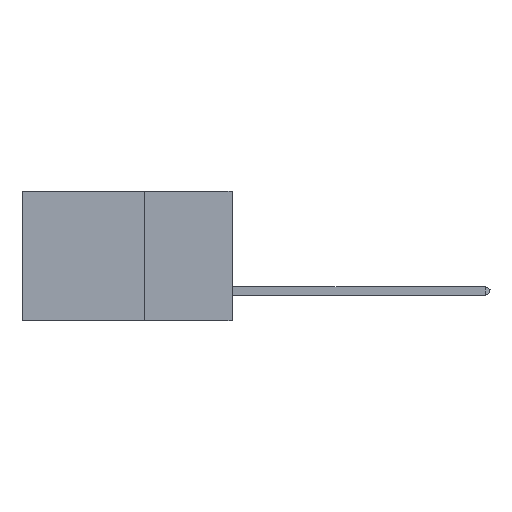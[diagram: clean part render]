
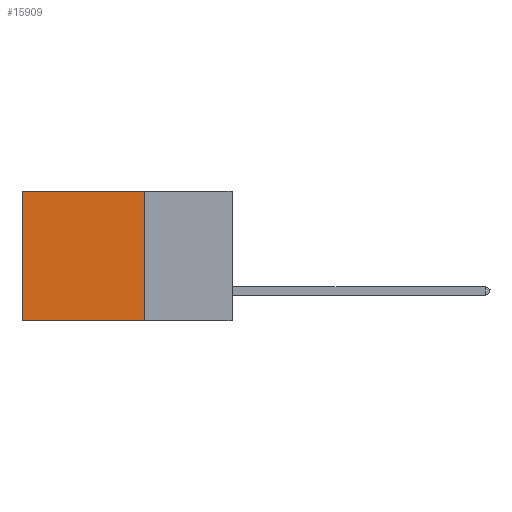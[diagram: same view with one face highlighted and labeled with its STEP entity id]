
A CAD part, left-side view. The second image highlights one B-rep face of the part: STEP entity #15909.
In plain terms, the highlighted planar face has unit normal (-1, 0, 0).
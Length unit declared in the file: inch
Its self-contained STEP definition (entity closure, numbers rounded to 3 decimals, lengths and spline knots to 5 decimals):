
#375 = DIRECTION ( 'NONE',  ( 0., 0., -1. ) ) ;
#440 = EDGE_CURVE ( 'NONE', #1478, #10378, #4758, .T. ) ;
#622 = ORIENTED_EDGE ( 'NONE', *, *, #9371, .F. ) ;
#645 = LINE ( 'NONE', #6478, #4033 ) ;
#1478 = VERTEX_POINT ( 'NONE', #11658 ) ;
#2903 = DIRECTION ( 'NONE',  ( 0., 0., -1. ) ) ;
#3101 = DIRECTION ( 'NONE',  ( 0., 1., 0. ) ) ;
#4033 = VECTOR ( 'NONE', #375, 39.37008 ) ;
#4150 = CARTESIAN_POINT ( 'NONE',  ( 0.2875, 0.25, 0. ) ) ;
#4238 = VERTEX_POINT ( 'NONE', #16393 ) ;
#4283 = DIRECTION ( 'NONE',  ( 0., 0., -1. ) ) ;
#4363 = VERTEX_POINT ( 'NONE', #14102 ) ;
#4745 = EDGE_CURVE ( 'NONE', #10378, #4363, #645, .T. ) ;
#4758 = LINE ( 'NONE', #4150, #15605 ) ;
#4925 = ORIENTED_EDGE ( 'NONE', *, *, #440, .T. ) ;
#4988 = VECTOR ( 'NONE', #2903, 39.37008 ) ;
#5394 = VECTOR ( 'NONE', #8800, 39.37008 ) ;
#5645 = CARTESIAN_POINT ( 'NONE',  ( 0.2875, 0.25, 0. ) ) ;
#6478 = CARTESIAN_POINT ( 'NONE',  ( 0.2875, 0.6, 0. ) ) ;
#8117 = CARTESIAN_POINT ( 'NONE',  ( 0.2875, 0.25, 0. ) ) ;
#8800 = DIRECTION ( 'NONE',  ( 0., 1., 0. ) ) ;
#9371 = EDGE_CURVE ( 'NONE', #4238, #4363, #10995, .T. ) ;
#9451 = CARTESIAN_POINT ( 'NONE',  ( 0.2875, 0.6, 0. ) ) ;
#9907 = ORIENTED_EDGE ( 'NONE', *, *, #14865, .F. ) ;
#10378 = VERTEX_POINT ( 'NONE', #9451 ) ;
#10818 = LINE ( 'NONE', #8117, #4988 ) ;
#10995 = LINE ( 'NONE', #16520, #5394 ) ;
#11658 = CARTESIAN_POINT ( 'NONE',  ( 0.2875, 0.25, 0. ) ) ;
#13304 = DIRECTION ( 'NONE',  ( 1., 0., 0. ) ) ;
#13931 = EDGE_LOOP ( 'NONE', ( #15402, #622, #9907, #4925 ) ) ;
#13989 = FACE_OUTER_BOUND ( 'NONE', #13931, .T. ) ;
#14102 = CARTESIAN_POINT ( 'NONE',  ( 0.2875, 0.6, -0.37 ) ) ;
#14865 = EDGE_CURVE ( 'NONE', #1478, #4238, #10818, .T. ) ;
#14943 = AXIS2_PLACEMENT_3D ( 'NONE', #5645, #13304, #4283 ) ;
#15402 = ORIENTED_EDGE ( 'NONE', *, *, #4745, .T. ) ;
#15605 = VECTOR ( 'NONE', #3101, 39.37008 ) ;
#15909 = ADVANCED_FACE ( 'NONE', ( #13989 ), #16014, .F. ) ;
#16014 = PLANE ( 'NONE',  #14943 ) ;
#16393 = CARTESIAN_POINT ( 'NONE',  ( 0.2875, 0.25, -0.37 ) ) ;
#16520 = CARTESIAN_POINT ( 'NONE',  ( 0.2875, 0.25, -0.37 ) ) ;
